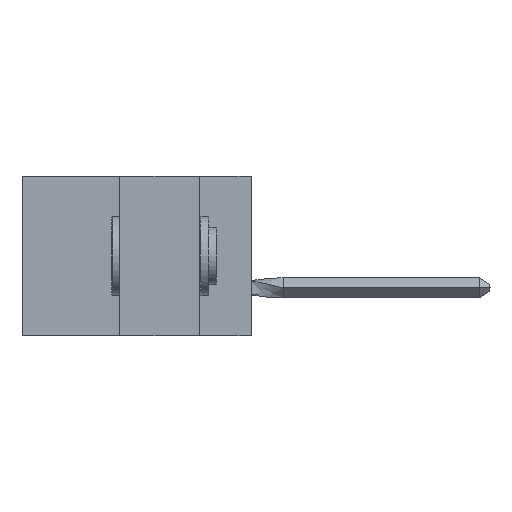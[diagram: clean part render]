
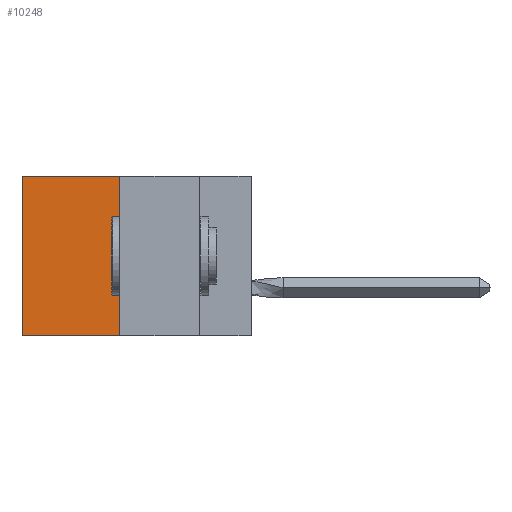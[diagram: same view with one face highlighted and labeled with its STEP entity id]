
A CAD part, left-side view. The second image highlights one B-rep face of the part: STEP entity #10248.
In plain terms, the highlighted planar face has unit normal (-1, 0, 0).
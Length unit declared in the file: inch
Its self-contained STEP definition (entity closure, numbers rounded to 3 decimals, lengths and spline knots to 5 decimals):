
#1444 = AXIS2_PLACEMENT_3D ( 'NONE', #15448, #17955, #26264 ) ;
#1576 = EDGE_CURVE ( 'NONE', #33450, #24265, #26282, .T. ) ;
#2050 = DIRECTION ( 'NONE',  ( 0., 1., 0. ) ) ;
#2534 = LINE ( 'NONE', #18802, #24726 ) ;
#3829 = EDGE_CURVE ( 'NONE', #31783, #14549, #2534, .T. ) ;
#6037 = CARTESIAN_POINT ( 'NONE',  ( 0.305, 0.413, -0.5 ) ) ;
#6140 = CARTESIAN_POINT ( 'NONE',  ( 0.305, 0.72, -0.5 ) ) ;
#6900 = PLANE ( 'NONE',  #1444 ) ;
#8332 = CARTESIAN_POINT ( 'NONE',  ( 0.305, 0.413, -0.5 ) ) ;
#10248 = ADVANCED_FACE ( 'NONE', ( #19451 ), #6900, .F. ) ;
#10565 = VECTOR ( 'NONE', #24744, 39.37008 ) ;
#10996 = EDGE_LOOP ( 'NONE', ( #24569, #16197, #30976, #33256 ) ) ;
#13950 = VECTOR ( 'NONE', #16949, 39.37008 ) ;
#14549 = VERTEX_POINT ( 'NONE', #6140 ) ;
#15448 = CARTESIAN_POINT ( 'NONE',  ( 0.305, 0.413, -0.5 ) ) ;
#16197 = ORIENTED_EDGE ( 'NONE', *, *, #3829, .F. ) ;
#16682 = EDGE_CURVE ( 'NONE', #24265, #14549, #16983, .T. ) ;
#16949 = DIRECTION ( 'NONE',  ( 0., 0., -1. ) ) ;
#16983 = LINE ( 'NONE', #28034, #33477 ) ;
#17955 = DIRECTION ( 'NONE',  ( 1., 0., 0. ) ) ;
#18802 = CARTESIAN_POINT ( 'NONE',  ( 0.305, 0.413, -0.5 ) ) ;
#19451 = FACE_OUTER_BOUND ( 'NONE', #10996, .T. ) ;
#19458 = CARTESIAN_POINT ( 'NONE',  ( 0.305, 0.413, 0. ) ) ;
#20241 = CARTESIAN_POINT ( 'NONE',  ( 0.305, 0.413, 0. ) ) ;
#22831 = DIRECTION ( 'NONE',  ( 0., 0., -1. ) ) ;
#24265 = VERTEX_POINT ( 'NONE', #35259 ) ;
#24569 = ORIENTED_EDGE ( 'NONE', *, *, #16682, .T. ) ;
#24726 = VECTOR ( 'NONE', #2050, 39.37008 ) ;
#24744 = DIRECTION ( 'NONE',  ( 0., 1., 0. ) ) ;
#26264 = DIRECTION ( 'NONE',  ( 0., 0., -1. ) ) ;
#26282 = LINE ( 'NONE', #19458, #10565 ) ;
#28034 = CARTESIAN_POINT ( 'NONE',  ( 0.305, 0.72, -0.5 ) ) ;
#28570 = EDGE_CURVE ( 'NONE', #33450, #31783, #30895, .T. ) ;
#30895 = LINE ( 'NONE', #8332, #13950 ) ;
#30976 = ORIENTED_EDGE ( 'NONE', *, *, #28570, .F. ) ;
#31783 = VERTEX_POINT ( 'NONE', #6037 ) ;
#33256 = ORIENTED_EDGE ( 'NONE', *, *, #1576, .T. ) ;
#33450 = VERTEX_POINT ( 'NONE', #20241 ) ;
#33477 = VECTOR ( 'NONE', #22831, 39.37008 ) ;
#35259 = CARTESIAN_POINT ( 'NONE',  ( 0.305, 0.72, 0. ) ) ;
